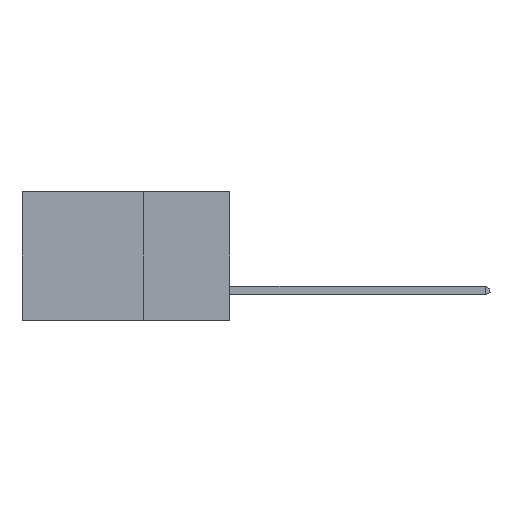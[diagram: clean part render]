
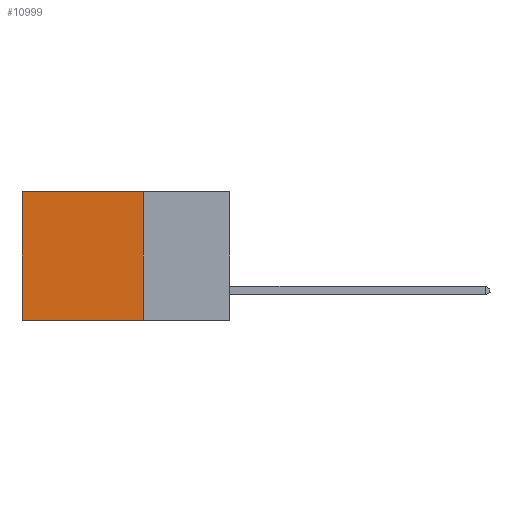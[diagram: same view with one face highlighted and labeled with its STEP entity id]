
A CAD part, left-side view. The second image highlights one B-rep face of the part: STEP entity #10999.
In plain terms, the highlighted planar face has unit normal (-1, 0, 0).
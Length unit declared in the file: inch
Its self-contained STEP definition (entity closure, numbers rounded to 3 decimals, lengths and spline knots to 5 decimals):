
#496 = DIRECTION ( 'NONE',  ( 0., 0., -1. ) ) ;
#1131 = VERTEX_POINT ( 'NONE', #8105 ) ;
#1770 = ORIENTED_EDGE ( 'NONE', *, *, #4984, .F. ) ;
#1842 = PLANE ( 'NONE',  #14445 ) ;
#2338 = VECTOR ( 'NONE', #8269, 39.37008 ) ;
#3811 = CARTESIAN_POINT ( 'NONE',  ( 0.298, 0.6, 0. ) ) ;
#4025 = LINE ( 'NONE', #3811, #22648 ) ;
#4565 = EDGE_CURVE ( 'NONE', #1131, #8347, #4025, .T. ) ;
#4984 = EDGE_CURVE ( 'NONE', #19730, #12887, #18485, .T. ) ;
#5425 = EDGE_CURVE ( 'NONE', #12887, #8347, #7107, .T. ) ;
#5600 = DIRECTION ( 'NONE',  ( 0., 0., -1. ) ) ;
#7107 = LINE ( 'NONE', #11598, #2338 ) ;
#7738 = ORIENTED_EDGE ( 'NONE', *, *, #5425, .F. ) ;
#8105 = CARTESIAN_POINT ( 'NONE',  ( 0.298, 0.6, 0. ) ) ;
#8269 = DIRECTION ( 'NONE',  ( 0., 1., 0. ) ) ;
#8347 = VERTEX_POINT ( 'NONE', #18112 ) ;
#9703 = CARTESIAN_POINT ( 'NONE',  ( 0.298, 0.25, -0.37 ) ) ;
#9823 = CARTESIAN_POINT ( 'NONE',  ( 0.298, 0.25, 0. ) ) ;
#10699 = VECTOR ( 'NONE', #11468, 39.37008 ) ;
#10824 = VECTOR ( 'NONE', #17483, 39.37008 ) ;
#10999 = ADVANCED_FACE ( 'NONE', ( #16190 ), #1842, .F. ) ;
#11468 = DIRECTION ( 'NONE',  ( 0., 0., -1. ) ) ;
#11598 = CARTESIAN_POINT ( 'NONE',  ( 0.298, 0.25, -0.37 ) ) ;
#11886 = CARTESIAN_POINT ( 'NONE',  ( 0.298, 0.25, 0. ) ) ;
#12887 = VERTEX_POINT ( 'NONE', #9703 ) ;
#14445 = AXIS2_PLACEMENT_3D ( 'NONE', #21054, #22844, #496 ) ;
#15573 = LINE ( 'NONE', #11886, #10824 ) ;
#16190 = FACE_OUTER_BOUND ( 'NONE', #18680, .T. ) ;
#17286 = EDGE_CURVE ( 'NONE', #19730, #1131, #15573, .T. ) ;
#17483 = DIRECTION ( 'NONE',  ( 0., 1., 0. ) ) ;
#17500 = ORIENTED_EDGE ( 'NONE', *, *, #4565, .T. ) ;
#17953 = ORIENTED_EDGE ( 'NONE', *, *, #17286, .T. ) ;
#18112 = CARTESIAN_POINT ( 'NONE',  ( 0.298, 0.6, -0.37 ) ) ;
#18485 = LINE ( 'NONE', #9823, #10699 ) ;
#18680 = EDGE_LOOP ( 'NONE', ( #17500, #7738, #1770, #17953 ) ) ;
#19730 = VERTEX_POINT ( 'NONE', #21948 ) ;
#21054 = CARTESIAN_POINT ( 'NONE',  ( 0.298, 0.25, 0. ) ) ;
#21948 = CARTESIAN_POINT ( 'NONE',  ( 0.298, 0.25, 0. ) ) ;
#22648 = VECTOR ( 'NONE', #5600, 39.37008 ) ;
#22844 = DIRECTION ( 'NONE',  ( 1., 0., 0. ) ) ;
